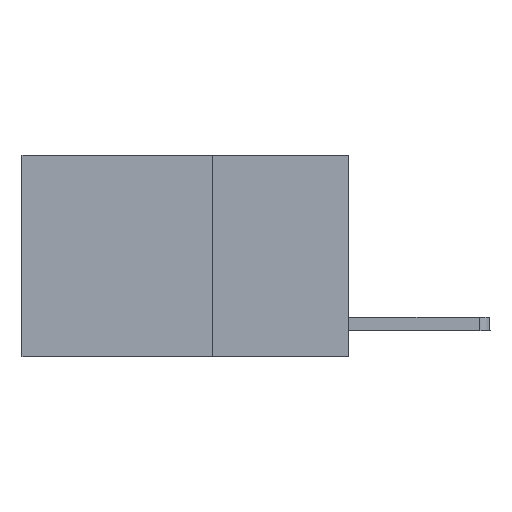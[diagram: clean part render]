
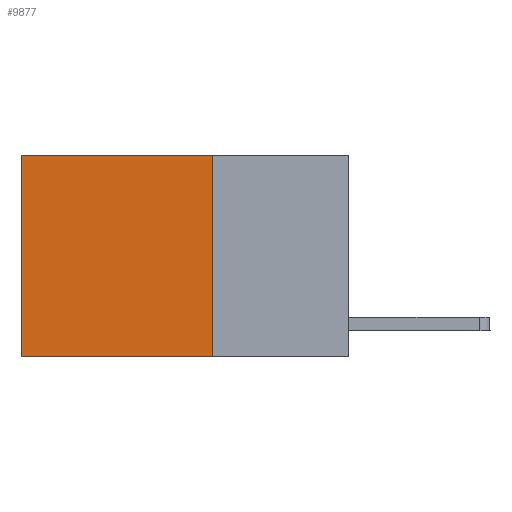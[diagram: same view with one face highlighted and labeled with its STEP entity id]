
A CAD part, left-side view. The second image highlights one B-rep face of the part: STEP entity #9877.
In plain terms, the highlighted planar face has unit normal (-1, 0, 0).
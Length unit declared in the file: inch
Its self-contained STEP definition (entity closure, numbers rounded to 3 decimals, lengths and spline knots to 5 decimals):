
#278 = LINE ( 'NONE', #9089, #10271 ) ;
#750 = DIRECTION ( 'NONE',  ( 0., 0., -1. ) ) ;
#1002 = CARTESIAN_POINT ( 'NONE',  ( 0.2625, 0.25, -0.37 ) ) ;
#1901 = VERTEX_POINT ( 'NONE', #8628 ) ;
#1965 = FACE_OUTER_BOUND ( 'NONE', #3804, .T. ) ;
#1999 = VECTOR ( 'NONE', #10839, 39.37008 ) ;
#2238 = VECTOR ( 'NONE', #750, 39.37008 ) ;
#2349 = EDGE_CURVE ( 'NONE', #5046, #8442, #7807, .T. ) ;
#2643 = DIRECTION ( 'NONE',  ( 1., 0., 0. ) ) ;
#3209 = CARTESIAN_POINT ( 'NONE',  ( 0.2625, 0.6, 0. ) ) ;
#3584 = DIRECTION ( 'NONE',  ( 0., 1., 0. ) ) ;
#3701 = LINE ( 'NONE', #10722, #1999 ) ;
#3804 = EDGE_LOOP ( 'NONE', ( #9079, #7952, #9419, #9776 ) ) ;
#4508 = PLANE ( 'NONE',  #5181 ) ;
#5046 = VERTEX_POINT ( 'NONE', #8787 ) ;
#5181 = AXIS2_PLACEMENT_3D ( 'NONE', #7928, #2643, #7062 ) ;
#6979 = LINE ( 'NONE', #10451, #7184 ) ;
#7062 = DIRECTION ( 'NONE',  ( 0., 0., -1. ) ) ;
#7184 = VECTOR ( 'NONE', #3584, 39.37008 ) ;
#7291 = EDGE_CURVE ( 'NONE', #7534, #1901, #3701, .T. ) ;
#7534 = VERTEX_POINT ( 'NONE', #3209 ) ;
#7807 = LINE ( 'NONE', #11158, #2238 ) ;
#7928 = CARTESIAN_POINT ( 'NONE',  ( 0.2625, 0.25, 0. ) ) ;
#7952 = ORIENTED_EDGE ( 'NONE', *, *, #10875, .F. ) ;
#8442 = VERTEX_POINT ( 'NONE', #1002 ) ;
#8628 = CARTESIAN_POINT ( 'NONE',  ( 0.2625, 0.6, -0.37 ) ) ;
#8787 = CARTESIAN_POINT ( 'NONE',  ( 0.2625, 0.25, 0. ) ) ;
#9079 = ORIENTED_EDGE ( 'NONE', *, *, #7291, .T. ) ;
#9089 = CARTESIAN_POINT ( 'NONE',  ( 0.2625, 0.25, 0. ) ) ;
#9419 = ORIENTED_EDGE ( 'NONE', *, *, #2349, .F. ) ;
#9776 = ORIENTED_EDGE ( 'NONE', *, *, #10890, .T. ) ;
#9877 = ADVANCED_FACE ( 'NONE', ( #1965 ), #4508, .F. ) ;
#10271 = VECTOR ( 'NONE', #10711, 39.37008 ) ;
#10451 = CARTESIAN_POINT ( 'NONE',  ( 0.2625, 0.25, -0.37 ) ) ;
#10711 = DIRECTION ( 'NONE',  ( 0., 1., 0. ) ) ;
#10722 = CARTESIAN_POINT ( 'NONE',  ( 0.2625, 0.6, 0. ) ) ;
#10839 = DIRECTION ( 'NONE',  ( 0., 0., -1. ) ) ;
#10875 = EDGE_CURVE ( 'NONE', #8442, #1901, #6979, .T. ) ;
#10890 = EDGE_CURVE ( 'NONE', #5046, #7534, #278, .T. ) ;
#11158 = CARTESIAN_POINT ( 'NONE',  ( 0.2625, 0.25, 0. ) ) ;
